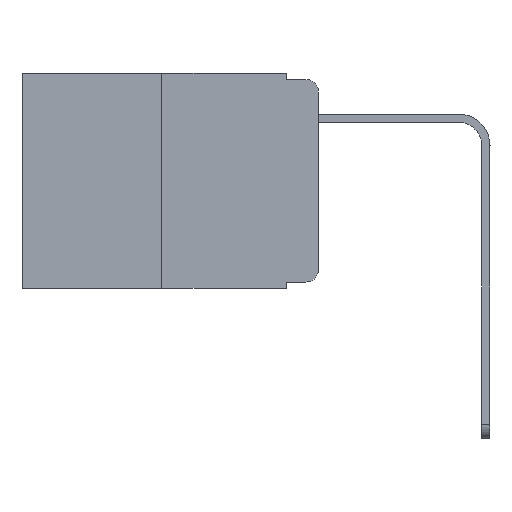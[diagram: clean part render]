
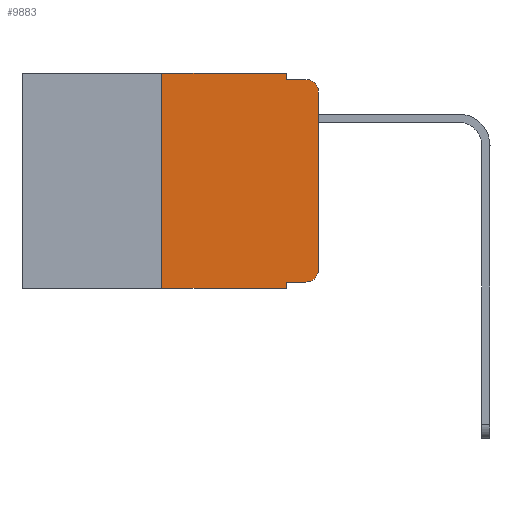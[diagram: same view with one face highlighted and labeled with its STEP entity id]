
A CAD part, left-side view. The second image highlights one B-rep face of the part: STEP entity #9883.
In plain terms, the highlighted planar face has unit normal (-1, 0, 0).
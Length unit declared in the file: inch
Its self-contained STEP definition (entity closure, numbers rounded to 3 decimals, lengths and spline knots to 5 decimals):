
#133 = FACE_OUTER_BOUND ( 'NONE', #9727, .T. ) ;
#228 = EDGE_CURVE ( 'NONE', #9324, #1101, #7003, .T. ) ;
#238 = ORIENTED_EDGE ( 'NONE', *, *, #228, .T. ) ;
#279 = CARTESIAN_POINT ( 'NONE',  ( 0., 0.051, -0.01 ) ) ;
#601 = ORIENTED_EDGE ( 'NONE', *, *, #1830, .T. ) ;
#879 = EDGE_CURVE ( 'NONE', #5047, #3138, #2032, .T. ) ;
#1056 = ORIENTED_EDGE ( 'NONE', *, *, #5743, .F. ) ;
#1101 = VERTEX_POINT ( 'NONE', #11065 ) ;
#1157 = VERTEX_POINT ( 'NONE', #8167 ) ;
#1328 = LINE ( 'NONE', #279, #9667 ) ;
#1569 = VERTEX_POINT ( 'NONE', #5335 ) ;
#1735 = CARTESIAN_POINT ( 'NONE',  ( 0., 0.473, 0. ) ) ;
#1830 = EDGE_CURVE ( 'NONE', #2640, #9324, #13118, .T. ) ;
#2032 = LINE ( 'NONE', #2878, #4237 ) ;
#2220 = ORIENTED_EDGE ( 'NONE', *, *, #10663, .T. ) ;
#2224 = AXIS2_PLACEMENT_3D ( 'NONE', #8727, #13951, #3201 ) ;
#2546 = CARTESIAN_POINT ( 'NONE',  ( 0., 0.051, -0.01 ) ) ;
#2632 = AXIS2_PLACEMENT_3D ( 'NONE', #4298, #11928, #7506 ) ;
#2640 = VERTEX_POINT ( 'NONE', #11348 ) ;
#2742 = ORIENTED_EDGE ( 'NONE', *, *, #5889, .T. ) ;
#2757 = CARTESIAN_POINT ( 'NONE',  ( 0., 0., -0.03 ) ) ;
#2787 = CARTESIAN_POINT ( 'NONE',  ( 0., 0.051, 0. ) ) ;
#2878 = CARTESIAN_POINT ( 'NONE',  ( 0., 0.25, 0. ) ) ;
#3024 = VECTOR ( 'NONE', #13546, 39.37008 ) ;
#3096 = CARTESIAN_POINT ( 'NONE',  ( 0., 0.051, -0.333 ) ) ;
#3138 = VERTEX_POINT ( 'NONE', #8269 ) ;
#3201 = DIRECTION ( 'NONE',  ( 0., 0., -1. ) ) ;
#3325 = DIRECTION ( 'NONE',  ( 0., 0., 1. ) ) ;
#3355 = LINE ( 'NONE', #11241, #7629 ) ;
#3470 = ORIENTED_EDGE ( 'NONE', *, *, #13897, .T. ) ;
#3695 = LINE ( 'NONE', #5672, #8476 ) ;
#4237 = VECTOR ( 'NONE', #13718, 39.37008 ) ;
#4278 = VERTEX_POINT ( 'NONE', #7998 ) ;
#4298 = CARTESIAN_POINT ( 'NONE',  ( 0., 0.473, 0. ) ) ;
#4433 = VECTOR ( 'NONE', #3325, 39.37008 ) ;
#4482 = DIRECTION ( 'NONE',  ( 0., 0., -1. ) ) ;
#4522 = DIRECTION ( 'NONE',  ( 0., -1., 0. ) ) ;
#4700 = DIRECTION ( 'NONE',  ( 0., -1., 0. ) ) ;
#4905 = LINE ( 'NONE', #2787, #3024 ) ;
#4964 = ORIENTED_EDGE ( 'NONE', *, *, #11188, .F. ) ;
#5047 = VERTEX_POINT ( 'NONE', #7551 ) ;
#5302 = VECTOR ( 'NONE', #11775, 39.37008 ) ;
#5335 = CARTESIAN_POINT ( 'NONE',  ( 0., 0.051, 0. ) ) ;
#5672 = CARTESIAN_POINT ( 'NONE',  ( 0., 0.473, -0.343 ) ) ;
#5743 = EDGE_CURVE ( 'NONE', #1569, #10179, #12072, .T. ) ;
#5815 = ORIENTED_EDGE ( 'NONE', *, *, #10582, .F. ) ;
#5889 = EDGE_CURVE ( 'NONE', #13346, #4278, #3355, .T. ) ;
#5938 = ORIENTED_EDGE ( 'NONE', *, *, #879, .F. ) ;
#6662 = LINE ( 'NONE', #1735, #5302 ) ;
#7003 = CIRCLE ( 'NONE', #10006, 0.02 ) ;
#7506 = DIRECTION ( 'NONE',  ( 0., 0., -1. ) ) ;
#7551 = CARTESIAN_POINT ( 'NONE',  ( 0., 0.25, -0.343 ) ) ;
#7625 = ORIENTED_EDGE ( 'NONE', *, *, #9709, .F. ) ;
#7629 = VECTOR ( 'NONE', #4700, 39.37008 ) ;
#7998 = CARTESIAN_POINT ( 'NONE',  ( 0., 0.02, -0.333 ) ) ;
#8167 = CARTESIAN_POINT ( 'NONE',  ( 0., 0.051, -0.343 ) ) ;
#8269 = CARTESIAN_POINT ( 'NONE',  ( 0., 0.25, 0. ) ) ;
#8300 = CIRCLE ( 'NONE', #2224, 0.02 ) ;
#8476 = VECTOR ( 'NONE', #4522, 39.37008 ) ;
#8727 = CARTESIAN_POINT ( 'NONE',  ( 0., 0.02, -0.313 ) ) ;
#9006 = CARTESIAN_POINT ( 'NONE',  ( 0., 0.051, 0. ) ) ;
#9324 = VERTEX_POINT ( 'NONE', #2757 ) ;
#9667 = VECTOR ( 'NONE', #12103, 39.37008 ) ;
#9709 = EDGE_CURVE ( 'NONE', #13346, #1157, #4905, .T. ) ;
#9727 = EDGE_LOOP ( 'NONE', ( #601, #238, #5815, #1056, #4964, #5938, #2220, #7625, #2742, #3470 ) ) ;
#9855 = VECTOR ( 'NONE', #10079, 39.37008 ) ;
#9883 = ADVANCED_FACE ( 'NONE', ( #133 ), #10828, .F. ) ;
#9909 = CARTESIAN_POINT ( 'NONE',  ( 0., 0.02, -0.03 ) ) ;
#10006 = AXIS2_PLACEMENT_3D ( 'NONE', #9909, #11012, #4482 ) ;
#10079 = DIRECTION ( 'NONE',  ( 0., 0., -1. ) ) ;
#10179 = VERTEX_POINT ( 'NONE', #2546 ) ;
#10582 = EDGE_CURVE ( 'NONE', #10179, #1101, #1328, .T. ) ;
#10663 = EDGE_CURVE ( 'NONE', #5047, #1157, #3695, .T. ) ;
#10828 = PLANE ( 'NONE',  #2632 ) ;
#11012 = DIRECTION ( 'NONE',  ( -1., 0., 0. ) ) ;
#11065 = CARTESIAN_POINT ( 'NONE',  ( 0., 0.02, -0.01 ) ) ;
#11188 = EDGE_CURVE ( 'NONE', #3138, #1569, #6662, .T. ) ;
#11241 = CARTESIAN_POINT ( 'NONE',  ( 0., 0.051, -0.333 ) ) ;
#11348 = CARTESIAN_POINT ( 'NONE',  ( 0., 0., -0.313 ) ) ;
#11775 = DIRECTION ( 'NONE',  ( 0., -1., 0. ) ) ;
#11928 = DIRECTION ( 'NONE',  ( 1., 0., 0. ) ) ;
#12072 = LINE ( 'NONE', #9006, #9855 ) ;
#12103 = DIRECTION ( 'NONE',  ( 0., -1., 0. ) ) ;
#13118 = LINE ( 'NONE', #13123, #4433 ) ;
#13123 = CARTESIAN_POINT ( 'NONE',  ( 0., 0., 0. ) ) ;
#13346 = VERTEX_POINT ( 'NONE', #3096 ) ;
#13546 = DIRECTION ( 'NONE',  ( 0., 0., -1. ) ) ;
#13718 = DIRECTION ( 'NONE',  ( 0., 0., 1. ) ) ;
#13897 = EDGE_CURVE ( 'NONE', #4278, #2640, #8300, .T. ) ;
#13951 = DIRECTION ( 'NONE',  ( -1., 0., 0. ) ) ;
